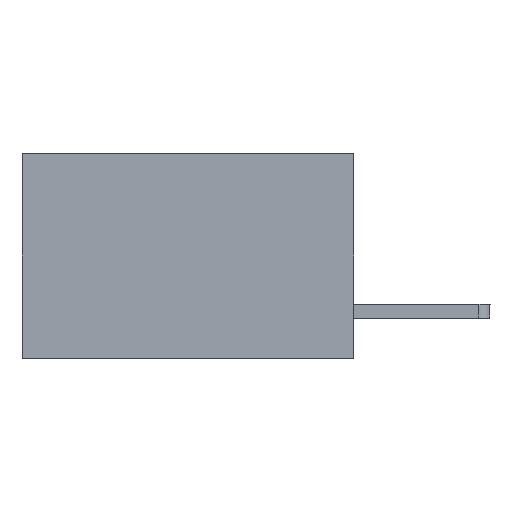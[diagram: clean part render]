
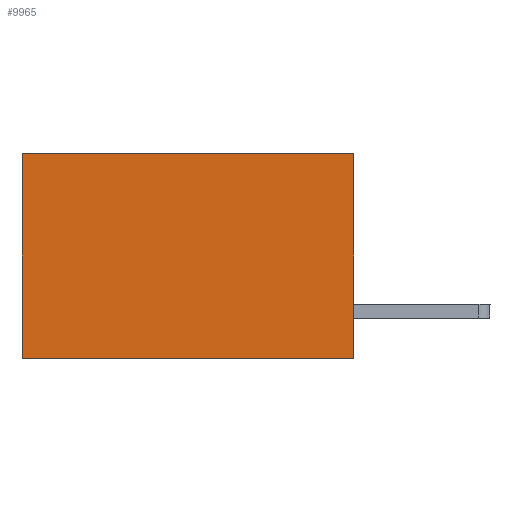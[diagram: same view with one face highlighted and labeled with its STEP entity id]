
A CAD part, left-side view. The second image highlights one B-rep face of the part: STEP entity #9965.
In plain terms, the highlighted planar face has unit normal (-1, 0, 0).
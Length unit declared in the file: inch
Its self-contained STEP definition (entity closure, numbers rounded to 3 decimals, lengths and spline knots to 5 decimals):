
#146 = VECTOR ( 'NONE', #2071, 39.37008 ) ;
#851 = LINE ( 'NONE', #2153, #3809 ) ;
#1189 = ORIENTED_EDGE ( 'NONE', *, *, #10803, .F. ) ;
#1314 = CARTESIAN_POINT ( 'NONE',  ( 0.2875, 0., 0. ) ) ;
#1327 = ORIENTED_EDGE ( 'NONE', *, *, #7131, .T. ) ;
#1383 = DIRECTION ( 'NONE',  ( 1., 0., 0. ) ) ;
#1545 = LINE ( 'NONE', #14566, #146 ) ;
#2071 = DIRECTION ( 'NONE',  ( 0., 0., -1. ) ) ;
#2153 = CARTESIAN_POINT ( 'NONE',  ( 0.2875, 0., 0. ) ) ;
#2898 = ORIENTED_EDGE ( 'NONE', *, *, #6218, .T. ) ;
#3126 = CARTESIAN_POINT ( 'NONE',  ( 0.2875, 0.6, -0.37 ) ) ;
#3809 = VECTOR ( 'NONE', #5980, 39.37008 ) ;
#3879 = DIRECTION ( 'NONE',  ( 0., 0., -1. ) ) ;
#5980 = DIRECTION ( 'NONE',  ( 0., 0., -1. ) ) ;
#6017 = CARTESIAN_POINT ( 'NONE',  ( 0.2875, 0., 0. ) ) ;
#6218 = EDGE_CURVE ( 'NONE', #12087, #12228, #1545, .T. ) ;
#6601 = PLANE ( 'NONE',  #14577 ) ;
#7131 = EDGE_CURVE ( 'NONE', #11341, #12087, #8880, .T. ) ;
#7233 = LINE ( 'NONE', #9407, #8431 ) ;
#7516 = DIRECTION ( 'NONE',  ( 0., 1., 0. ) ) ;
#7676 = EDGE_LOOP ( 'NONE', ( #2898, #1189, #7763, #1327 ) ) ;
#7763 = ORIENTED_EDGE ( 'NONE', *, *, #12895, .F. ) ;
#7916 = DIRECTION ( 'NONE',  ( 0., 1., 0. ) ) ;
#8156 = CARTESIAN_POINT ( 'NONE',  ( 0.2875, 0., 0. ) ) ;
#8431 = VECTOR ( 'NONE', #7916, 39.37008 ) ;
#8880 = LINE ( 'NONE', #1314, #13824 ) ;
#9063 = VERTEX_POINT ( 'NONE', #12524 ) ;
#9407 = CARTESIAN_POINT ( 'NONE',  ( 0.2875, 0., -0.37 ) ) ;
#9965 = ADVANCED_FACE ( 'NONE', ( #15758 ), #6601, .F. ) ;
#10803 = EDGE_CURVE ( 'NONE', #9063, #12228, #7233, .T. ) ;
#11341 = VERTEX_POINT ( 'NONE', #6017 ) ;
#12087 = VERTEX_POINT ( 'NONE', #12179 ) ;
#12179 = CARTESIAN_POINT ( 'NONE',  ( 0.2875, 0.6, 0. ) ) ;
#12228 = VERTEX_POINT ( 'NONE', #3126 ) ;
#12524 = CARTESIAN_POINT ( 'NONE',  ( 0.2875, 0., -0.37 ) ) ;
#12895 = EDGE_CURVE ( 'NONE', #11341, #9063, #851, .T. ) ;
#13824 = VECTOR ( 'NONE', #7516, 39.37008 ) ;
#14566 = CARTESIAN_POINT ( 'NONE',  ( 0.2875, 0.6, 0. ) ) ;
#14577 = AXIS2_PLACEMENT_3D ( 'NONE', #8156, #1383, #3879 ) ;
#15758 = FACE_OUTER_BOUND ( 'NONE', #7676, .T. ) ;
